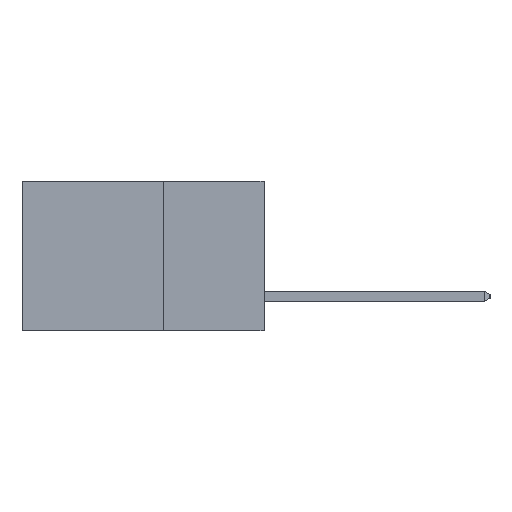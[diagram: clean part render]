
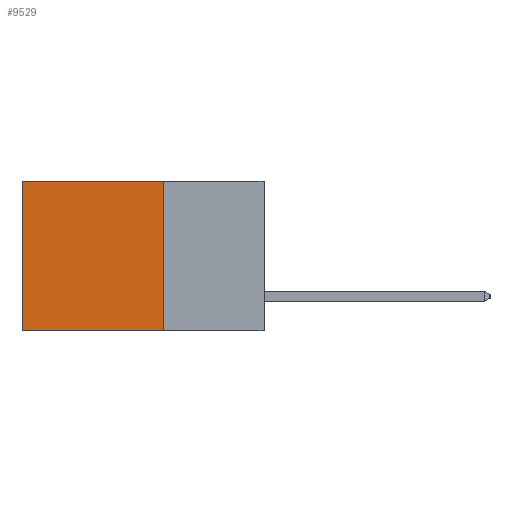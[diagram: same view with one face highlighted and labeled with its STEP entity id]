
A CAD part, left-side view. The second image highlights one B-rep face of the part: STEP entity #9529.
In plain terms, the highlighted planar face has unit normal (-1, 0, 0).
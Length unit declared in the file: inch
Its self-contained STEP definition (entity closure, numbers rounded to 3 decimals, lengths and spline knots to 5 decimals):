
#5 = EDGE_CURVE ( 'NONE', #1247, #7258, #10774, .T. ) ;
#654 = EDGE_LOOP ( 'NONE', ( #1520, #1547, #1563, #1653 ) ) ;
#1247 = VERTEX_POINT ( 'NONE', #10573 ) ;
#1520 = ORIENTED_EDGE ( 'NONE', *, *, #8662, .T. ) ;
#1547 = ORIENTED_EDGE ( 'NONE', *, *, #5, .F. ) ;
#1563 = ORIENTED_EDGE ( 'NONE', *, *, #3562, .F. ) ;
#1653 = ORIENTED_EDGE ( 'NONE', *, *, #3514, .T. ) ;
#1747 = DIRECTION ( 'NONE',  ( 0., 0., -1. ) ) ;
#1833 = CARTESIAN_POINT ( 'NONE',  ( 0.2615, 0.25, -0.37 ) ) ;
#2169 = CARTESIAN_POINT ( 'NONE',  ( 0.2615, 0.6, 0. ) ) ;
#2234 = DIRECTION ( 'NONE',  ( 0., 0., -1. ) ) ;
#2249 = DIRECTION ( 'NONE',  ( 1., 0., 0. ) ) ;
#2259 = CARTESIAN_POINT ( 'NONE',  ( 0.2615, 0.25, -0.37 ) ) ;
#2387 = PLANE ( 'NONE',  #2778 ) ;
#2443 = VECTOR ( 'NONE', #2729, 39.37008 ) ;
#2528 = VECTOR ( 'NONE', #10092, 39.37008 ) ;
#2638 = CARTESIAN_POINT ( 'NONE',  ( 0.2615, 0.25, 0. ) ) ;
#2729 = DIRECTION ( 'NONE',  ( 0., 1., 0. ) ) ;
#2778 = AXIS2_PLACEMENT_3D ( 'NONE', #2259, #2249, #2234 ) ;
#3331 = CARTESIAN_POINT ( 'NONE',  ( 0.2615, 0.25, 0. ) ) ;
#3514 = EDGE_CURVE ( 'NONE', #9323, #9535, #10725, .T. ) ;
#3562 = EDGE_CURVE ( 'NONE', #9323, #1247, #6233, .T. ) ;
#3595 = FACE_OUTER_BOUND ( 'NONE', #654, .T. ) ;
#3989 = VECTOR ( 'NONE', #1747, 39.37008 ) ;
#5883 = CARTESIAN_POINT ( 'NONE',  ( 0.2615, 0.6, -0.37 ) ) ;
#6233 = LINE ( 'NONE', #1833, #3989 ) ;
#6242 = DIRECTION ( 'NONE',  ( 0., 0., -1. ) ) ;
#6350 = CARTESIAN_POINT ( 'NONE',  ( 0.2615, 0.6, -0.37 ) ) ;
#7258 = VERTEX_POINT ( 'NONE', #5883 ) ;
#8662 = EDGE_CURVE ( 'NONE', #9535, #7258, #9990, .T. ) ;
#9323 = VERTEX_POINT ( 'NONE', #3331 ) ;
#9529 = ADVANCED_FACE ( 'NONE', ( #3595 ), #2387, .F. ) ;
#9535 = VERTEX_POINT ( 'NONE', #2169 ) ;
#9542 = VECTOR ( 'NONE', #6242, 39.37008 ) ;
#9791 = CARTESIAN_POINT ( 'NONE',  ( 0.2615, 0.25, -0.37 ) ) ;
#9990 = LINE ( 'NONE', #6350, #9542 ) ;
#10092 = DIRECTION ( 'NONE',  ( 0., 1., 0. ) ) ;
#10573 = CARTESIAN_POINT ( 'NONE',  ( 0.2615, 0.25, -0.37 ) ) ;
#10725 = LINE ( 'NONE', #2638, #2443 ) ;
#10774 = LINE ( 'NONE', #9791, #2528 ) ;
